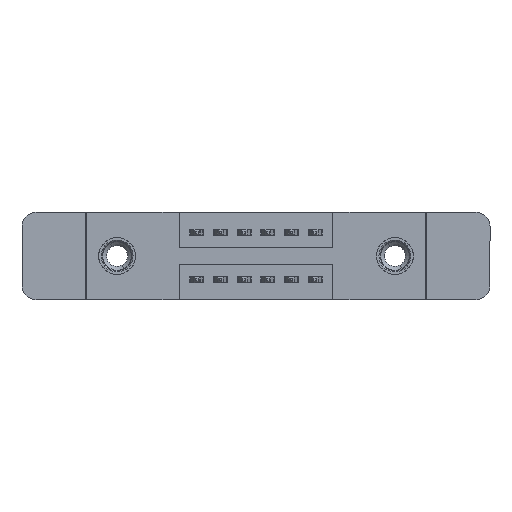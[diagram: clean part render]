
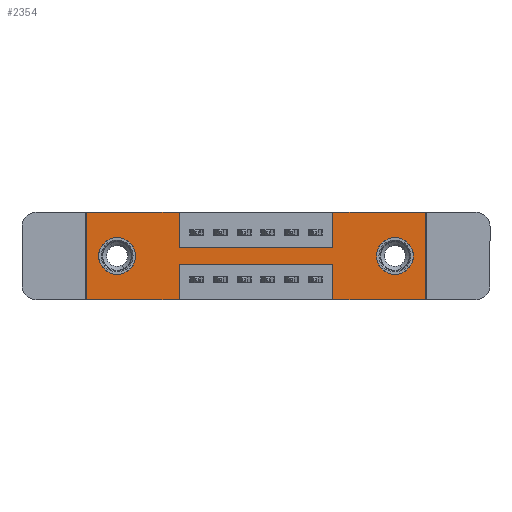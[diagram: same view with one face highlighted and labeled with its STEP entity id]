
A CAD part, front view. The second image highlights one B-rep face of the part: STEP entity #2354.
In plain terms, the highlighted planar face has unit normal (0, -1, 0).
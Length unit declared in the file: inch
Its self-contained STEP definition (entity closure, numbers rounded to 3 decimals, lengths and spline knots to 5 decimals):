
#143 = CARTESIAN_POINT ( 'NONE',  ( 0., 0., 0. ) ) ;
#230 = VERTEX_POINT ( 'NONE', #143 ) ;
#326 = CARTESIAN_POINT ( 'NONE',  ( 1.435, 0., -0.37 ) ) ;
#341 = EDGE_CURVE ( 'NONE', #230, #4790, #2258, .T. ) ;
#396 = CARTESIAN_POINT ( 'NONE',  ( 0.3925, 0., -0.37 ) ) ;
#493 = LINE ( 'NONE', #8059, #7384 ) ;
#551 = CARTESIAN_POINT ( 'NONE',  ( 0.13, 0., -0.107 ) ) ;
#605 = DIRECTION ( 'NONE',  ( 0., 1., 0. ) ) ;
#616 = EDGE_CURVE ( 'NONE', #4238, #6219, #13648, .T. ) ;
#646 = PLANE ( 'NONE',  #6110 ) ;
#653 = DIRECTION ( 'NONE',  ( 0., 0., -1. ) ) ;
#684 = AXIS2_PLACEMENT_3D ( 'NONE', #8527, #7327, #5171 ) ;
#695 = DIRECTION ( 'NONE',  ( 0., 0., -1. ) ) ;
#716 = VECTOR ( 'NONE', #6824, 39.37008 ) ;
#732 = AXIS2_PLACEMENT_3D ( 'NONE', #10737, #4841, #8293 ) ;
#788 = CARTESIAN_POINT ( 'NONE',  ( 0., 0., -0.37 ) ) ;
#803 = ORIENTED_EDGE ( 'NONE', *, *, #8307, .F. ) ;
#841 = CARTESIAN_POINT ( 'NONE',  ( 1.305, 0., -0.185 ) ) ;
#859 = LINE ( 'NONE', #10903, #9363 ) ;
#928 = EDGE_CURVE ( 'NONE', #1338, #8566, #11184, .T. ) ;
#1052 = LINE ( 'NONE', #2601, #12452 ) ;
#1168 = EDGE_CURVE ( 'NONE', #9412, #1671, #10627, .T. ) ;
#1181 = VERTEX_POINT ( 'NONE', #10227 ) ;
#1210 = VECTOR ( 'NONE', #5944, 39.37008 ) ;
#1338 = VERTEX_POINT ( 'NONE', #14201 ) ;
#1520 = CARTESIAN_POINT ( 'NONE',  ( 0.3925, 0., -0.22 ) ) ;
#1671 = VERTEX_POINT ( 'NONE', #11321 ) ;
#1704 = DIRECTION ( 'NONE',  ( 1., 0., 0. ) ) ;
#2178 = VERTEX_POINT ( 'NONE', #11927 ) ;
#2228 = FACE_BOUND ( 'NONE', #7922, .T. ) ;
#2258 = LINE ( 'NONE', #12858, #1210 ) ;
#2295 = VERTEX_POINT ( 'NONE', #4756 ) ;
#2354 = ADVANCED_FACE ( 'NONE', ( #2228, #13297, #7912 ), #646, .T. ) ;
#2476 = CARTESIAN_POINT ( 'NONE',  ( 0.3925, 0., -0.22 ) ) ;
#2588 = ORIENTED_EDGE ( 'NONE', *, *, #341, .F. ) ;
#2601 = CARTESIAN_POINT ( 'NONE',  ( 0., 0., 0. ) ) ;
#2662 = CARTESIAN_POINT ( 'NONE',  ( 0.3925, 0., 0. ) ) ;
#2696 = CARTESIAN_POINT ( 'NONE',  ( 1.305, 0., -0.185 ) ) ;
#2721 = CARTESIAN_POINT ( 'NONE',  ( 1.0425, 0., 0. ) ) ;
#2729 = DIRECTION ( 'NONE',  ( 0., 0., -1. ) ) ;
#2804 = CIRCLE ( 'NONE', #8973, 0.078 ) ;
#2925 = ORIENTED_EDGE ( 'NONE', *, *, #4572, .T. ) ;
#3122 = CARTESIAN_POINT ( 'NONE',  ( 0.13, 0., -0.263 ) ) ;
#3189 = DIRECTION ( 'NONE',  ( 0., 0., -1. ) ) ;
#3234 = CARTESIAN_POINT ( 'NONE',  ( 1.0425, 0., -0.15 ) ) ;
#3344 = VECTOR ( 'NONE', #7108, 39.37008 ) ;
#3362 = CIRCLE ( 'NONE', #684, 0.078 ) ;
#3641 = EDGE_CURVE ( 'NONE', #6219, #1338, #9687, .T. ) ;
#3651 = VERTEX_POINT ( 'NONE', #3122 ) ;
#3789 = DIRECTION ( 'NONE',  ( 0., 0., 1. ) ) ;
#3841 = LINE ( 'NONE', #396, #10420 ) ;
#3857 = DIRECTION ( 'NONE',  ( 0., 0., 1. ) ) ;
#3880 = EDGE_LOOP ( 'NONE', ( #4227, #803, #6640, #5564, #6687, #9602, #14059, #14347, #10026, #2588, #6264, #14007 ) ) ;
#3921 = CARTESIAN_POINT ( 'NONE',  ( 0., 0., -0.37 ) ) ;
#4227 = ORIENTED_EDGE ( 'NONE', *, *, #13744, .F. ) ;
#4238 = VERTEX_POINT ( 'NONE', #11854 ) ;
#4529 = ORIENTED_EDGE ( 'NONE', *, *, #12180, .T. ) ;
#4572 = EDGE_CURVE ( 'NONE', #1181, #2178, #12548, .T. ) ;
#4672 = LINE ( 'NONE', #2476, #10373 ) ;
#4756 = CARTESIAN_POINT ( 'NONE',  ( 0.3925, 0., -0.15 ) ) ;
#4790 = VERTEX_POINT ( 'NONE', #2662 ) ;
#4841 = DIRECTION ( 'NONE',  ( 0., 1., 0. ) ) ;
#5049 = VECTOR ( 'NONE', #6528, 39.37008 ) ;
#5171 = DIRECTION ( 'NONE',  ( 0., 0., 1. ) ) ;
#5564 = ORIENTED_EDGE ( 'NONE', *, *, #3641, .F. ) ;
#5673 = CARTESIAN_POINT ( 'NONE',  ( 1.0425, 0., -0.22 ) ) ;
#5944 = DIRECTION ( 'NONE',  ( 1., 0., 0. ) ) ;
#5966 = CARTESIAN_POINT ( 'NONE',  ( 0.3925, 0., 0. ) ) ;
#6110 = AXIS2_PLACEMENT_3D ( 'NONE', #3921, #14207, #695 ) ;
#6219 = VERTEX_POINT ( 'NONE', #326 ) ;
#6264 = ORIENTED_EDGE ( 'NONE', *, *, #13116, .F. ) ;
#6370 = CIRCLE ( 'NONE', #732, 0.078 ) ;
#6528 = DIRECTION ( 'NONE',  ( -1., 0., 0. ) ) ;
#6530 = CARTESIAN_POINT ( 'NONE',  ( 1.0425, 0., -0.37 ) ) ;
#6640 = ORIENTED_EDGE ( 'NONE', *, *, #928, .F. ) ;
#6687 = ORIENTED_EDGE ( 'NONE', *, *, #616, .F. ) ;
#6824 = DIRECTION ( 'NONE',  ( 0., 0., 1. ) ) ;
#7108 = DIRECTION ( 'NONE',  ( 0., 0., -1. ) ) ;
#7139 = DIRECTION ( 'NONE',  ( -1., 0., 0. ) ) ;
#7327 = DIRECTION ( 'NONE',  ( 0., 1., 0. ) ) ;
#7384 = VECTOR ( 'NONE', #12673, 39.37008 ) ;
#7407 = VECTOR ( 'NONE', #3857, 39.37008 ) ;
#7441 = EDGE_CURVE ( 'NONE', #3651, #11570, #3362, .T. ) ;
#7912 = FACE_OUTER_BOUND ( 'NONE', #3880, .T. ) ;
#7922 = EDGE_LOOP ( 'NONE', ( #2925, #10419 ) ) ;
#7929 = EDGE_CURVE ( 'NONE', #8821, #13347, #12098, .T. ) ;
#8059 = CARTESIAN_POINT ( 'NONE',  ( 0., 0., 0. ) ) ;
#8293 = DIRECTION ( 'NONE',  ( 0., 0., 1. ) ) ;
#8307 = EDGE_CURVE ( 'NONE', #8566, #8484, #4672, .T. ) ;
#8484 = VERTEX_POINT ( 'NONE', #1520 ) ;
#8527 = CARTESIAN_POINT ( 'NONE',  ( 0.13, 0., -0.185 ) ) ;
#8566 = VERTEX_POINT ( 'NONE', #5673 ) ;
#8821 = VERTEX_POINT ( 'NONE', #3234 ) ;
#8973 = AXIS2_PLACEMENT_3D ( 'NONE', #2696, #605, #653 ) ;
#8989 = AXIS2_PLACEMENT_3D ( 'NONE', #841, #11101, #3189 ) ;
#9363 = VECTOR ( 'NONE', #1704, 39.37008 ) ;
#9412 = VERTEX_POINT ( 'NONE', #14532 ) ;
#9544 = CARTESIAN_POINT ( 'NONE',  ( 1.0425, 0., 0. ) ) ;
#9602 = ORIENTED_EDGE ( 'NONE', *, *, #14475, .F. ) ;
#9687 = LINE ( 'NONE', #788, #5049 ) ;
#10026 = ORIENTED_EDGE ( 'NONE', *, *, #13236, .F. ) ;
#10227 = CARTESIAN_POINT ( 'NONE',  ( 1.305, 0., -0.107 ) ) ;
#10373 = VECTOR ( 'NONE', #7139, 39.37008 ) ;
#10419 = ORIENTED_EDGE ( 'NONE', *, *, #13357, .T. ) ;
#10420 = VECTOR ( 'NONE', #2729, 39.37008 ) ;
#10431 = DIRECTION ( 'NONE',  ( -1., 0., 0. ) ) ;
#10627 = LINE ( 'NONE', #13286, #13167 ) ;
#10737 = CARTESIAN_POINT ( 'NONE',  ( 0.13, 0., -0.185 ) ) ;
#10903 = CARTESIAN_POINT ( 'NONE',  ( 0.3925, 0., -0.15 ) ) ;
#11101 = DIRECTION ( 'NONE',  ( 0., 1., 0. ) ) ;
#11184 = LINE ( 'NONE', #6530, #716 ) ;
#11321 = CARTESIAN_POINT ( 'NONE',  ( 0., 0., -0.37 ) ) ;
#11350 = CARTESIAN_POINT ( 'NONE',  ( 1.435, 0., 0. ) ) ;
#11570 = VERTEX_POINT ( 'NONE', #551 ) ;
#11854 = CARTESIAN_POINT ( 'NONE',  ( 1.435, 0., 0. ) ) ;
#11927 = CARTESIAN_POINT ( 'NONE',  ( 1.305, 0., -0.263 ) ) ;
#12098 = LINE ( 'NONE', #2721, #7407 ) ;
#12180 = EDGE_CURVE ( 'NONE', #11570, #3651, #6370, .T. ) ;
#12452 = VECTOR ( 'NONE', #3789, 39.37008 ) ;
#12548 = CIRCLE ( 'NONE', #8989, 0.078 ) ;
#12673 = DIRECTION ( 'NONE',  ( 1., 0., 0. ) ) ;
#12858 = CARTESIAN_POINT ( 'NONE',  ( 0., 0., 0. ) ) ;
#13098 = ORIENTED_EDGE ( 'NONE', *, *, #7441, .T. ) ;
#13116 = EDGE_CURVE ( 'NONE', #1671, #230, #1052, .T. ) ;
#13167 = VECTOR ( 'NONE', #10431, 39.37008 ) ;
#13236 = EDGE_CURVE ( 'NONE', #4790, #2295, #13682, .T. ) ;
#13286 = CARTESIAN_POINT ( 'NONE',  ( 0., 0., -0.37 ) ) ;
#13297 = FACE_BOUND ( 'NONE', #13313, .T. ) ;
#13313 = EDGE_LOOP ( 'NONE', ( #4529, #13098 ) ) ;
#13347 = VERTEX_POINT ( 'NONE', #9544 ) ;
#13357 = EDGE_CURVE ( 'NONE', #2178, #1181, #2804, .T. ) ;
#13648 = LINE ( 'NONE', #11350, #14591 ) ;
#13682 = LINE ( 'NONE', #5966, #3344 ) ;
#13744 = EDGE_CURVE ( 'NONE', #8484, #9412, #3841, .T. ) ;
#13890 = EDGE_CURVE ( 'NONE', #2295, #8821, #859, .T. ) ;
#14007 = ORIENTED_EDGE ( 'NONE', *, *, #1168, .F. ) ;
#14059 = ORIENTED_EDGE ( 'NONE', *, *, #7929, .F. ) ;
#14201 = CARTESIAN_POINT ( 'NONE',  ( 1.0425, 0., -0.37 ) ) ;
#14207 = DIRECTION ( 'NONE',  ( 0., -1., 0. ) ) ;
#14347 = ORIENTED_EDGE ( 'NONE', *, *, #13890, .F. ) ;
#14475 = EDGE_CURVE ( 'NONE', #13347, #4238, #493, .T. ) ;
#14532 = CARTESIAN_POINT ( 'NONE',  ( 0.3925, 0., -0.37 ) ) ;
#14591 = VECTOR ( 'NONE', #14745, 39.37008 ) ;
#14745 = DIRECTION ( 'NONE',  ( 0., 0., -1. ) ) ;
